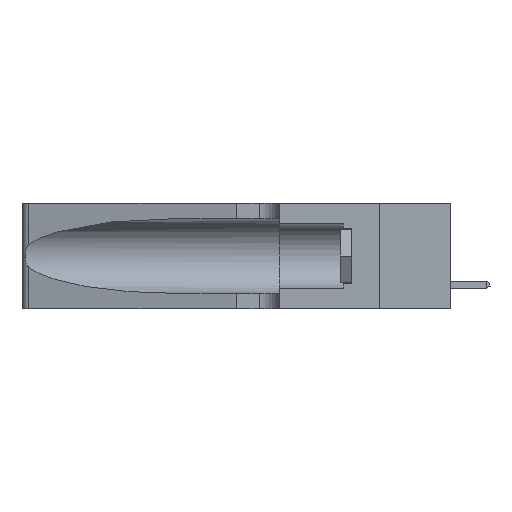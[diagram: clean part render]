
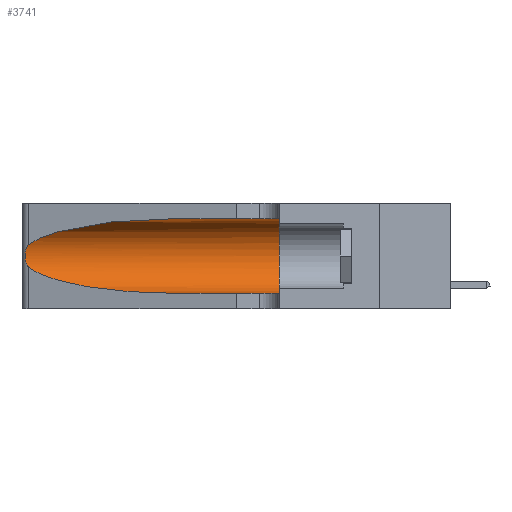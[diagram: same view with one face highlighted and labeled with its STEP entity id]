
A CAD part, left-side view. The second image highlights one B-rep face of the part: STEP entity #3741.
In plain terms, the highlighted cylindrical face has radius 3.308 mm (diameter 6.617 mm), a partial arc.
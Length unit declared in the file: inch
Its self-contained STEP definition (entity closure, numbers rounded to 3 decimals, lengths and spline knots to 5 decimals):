
#56 = CARTESIAN_POINT ( 'NONE',  ( 0.18966, 0.96281, 0.05475 ) ) ;
#865 = CARTESIAN_POINT ( 'NONE',  ( 0.26018, 1.23835, 0.19895 ) ) ;
#2405 = VERTEX_POINT ( 'NONE', #3868 ) ;
#3090 = VERTEX_POINT ( 'NONE', #22199 ) ;
#3415 = VERTEX_POINT ( 'NONE', #16453 ) ;
#3493 = CARTESIAN_POINT ( 'NONE',  ( 0.1305, 0.72297, 0.31525 ) ) ;
#3563 = EDGE_LOOP ( 'NONE', ( #20343, #20942, #22353, #11715, #9644, #24472 ) ) ;
#3741 = ADVANCED_FACE ( 'NONE', ( #6569 ), #15394, .F. ) ;
#3868 = CARTESIAN_POINT ( 'NONE',  ( 0.1305, 0.72297, 0.05475 ) ) ;
#3903 = CARTESIAN_POINT ( 'NONE',  ( 0.1305, 1.61858, 0.05475 ) ) ;
#4370 = CARTESIAN_POINT ( 'NONE',  ( 0.25787, 1.23484, 0.2124 ) ) ;
#4598 = DIRECTION ( 'NONE',  ( 0., -1., 0. ) ) ;
#4611 = VERTEX_POINT ( 'NONE', #9535 ) ;
#5170 = EDGE_CURVE ( 'NONE', #4611, #8581, #16346, .T. ) ;
#5773 = DIRECTION ( 'NONE',  ( 0., -1., 0. ) ) ;
#6014 = EDGE_CURVE ( 'NONE', #4611, #3415, #7759, .T. ) ;
#6287 = CARTESIAN_POINT ( 'NONE',  ( 0.25555, 1.22993, 0.14849 ) ) ;
#6569 = FACE_OUTER_BOUND ( 'NONE', #3563, .T. ) ;
#7571 = EDGE_CURVE ( 'NONE', #8581, #3090, #8627, .T. ) ;
#7658 = AXIS2_PLACEMENT_3D ( 'NONE', #19523, #15509, #13701 ) ;
#7759 = LINE ( 'NONE', #19672, #21714 ) ;
#7877 = CARTESIAN_POINT ( 'NONE',  ( 0.2373, 1.15595, 0.08982 ) ) ;
#8350 = CARTESIAN_POINT ( 'NONE',  ( 0.25854, 1.2359, 0.20912 ) ) ;
#8578 = CARTESIAN_POINT ( 'NONE',  ( 0.1305, 0.35, 0.185 ) ) ;
#8581 = VERTEX_POINT ( 'NONE', #15327 ) ;
#8627 = B_SPLINE_CURVE_WITH_KNOTS ( 'NONE', 3,
 ( #12137, #13804, #17693, #4370, #8350, #865, #23260, #11877, #17789, #10023, #13894, #19533, #6287, #10181 ),
 .UNSPECIFIED., .F., .F.,
 ( 4, 2, 2, 2, 2, 2, 4 ),
 ( 0., 0.00027, 0.00053, 0.00107, 0.0016, 0.00187, 0.00214 ),
 .UNSPECIFIED. ) ;
#8733 = DIRECTION ( 'NONE',  ( 0., 0., 1. ) ) ;
#9535 = CARTESIAN_POINT ( 'NONE',  ( 0.1305, 0.72297, 0.31525 ) ) ;
#9644 = ORIENTED_EDGE ( 'NONE', *, *, #20169, .F. ) ;
#10023 = CARTESIAN_POINT ( 'NONE',  ( 0.25856, 1.23593, 0.16098 ) ) ;
#10181 = CARTESIAN_POINT ( 'NONE',  ( 0.25487, 1.22718, 0.14631 ) ) ;
#10834 = EDGE_CURVE ( 'NONE', #3090, #2405, #15575, .T. ) ;
#11422 = EDGE_CURVE ( 'NONE', #2405, #16798, #13759, .T. ) ;
#11657 = CARTESIAN_POINT ( 'NONE',  ( 0.1305, 0.72297, 0.05475 ) ) ;
#11715 = ORIENTED_EDGE ( 'NONE', *, *, #11422, .T. ) ;
#11877 = CARTESIAN_POINT ( 'NONE',  ( 0.26075, 1.23896, 0.178 ) ) ;
#11966 = AXIS2_PLACEMENT_3D ( 'NONE', #8578, #12612, #8733 ) ;
#12137 = CARTESIAN_POINT ( 'NONE',  ( 0.25487, 1.22718, 0.22369 ) ) ;
#12612 = DIRECTION ( 'NONE',  ( 0., 1., 0. ) ) ;
#13701 = DIRECTION ( 'NONE',  ( 0., 0., -1. ) ) ;
#13759 = LINE ( 'NONE', #3903, #23540 ) ;
#13804 = CARTESIAN_POINT ( 'NONE',  ( 0.25555, 1.22994, 0.2215 ) ) ;
#13894 = CARTESIAN_POINT ( 'NONE',  ( 0.25789, 1.23486, 0.15765 ) ) ;
#15252 = CARTESIAN_POINT ( 'NONE',  ( 0.25487, 1.22718, 0.22369 ) ) ;
#15307 = CARTESIAN_POINT ( 'NONE',  ( 0.25487, 1.22718, 0.14631 ) ) ;
#15327 = CARTESIAN_POINT ( 'NONE',  ( 0.25487, 1.22718, 0.22369 ) ) ;
#15394 = CYLINDRICAL_SURFACE ( 'NONE', #7658, 0.13025 ) ;
#15423 = CARTESIAN_POINT ( 'NONE',  ( 0.2373, 1.15595, 0.28018 ) ) ;
#15509 = DIRECTION ( 'NONE',  ( 0., -1., 0. ) ) ;
#15575 =( BOUNDED_CURVE ( )  B_SPLINE_CURVE ( 3, ( #15307, #7877, #56, #11657 ),
 .UNSPECIFIED., .F., .T. ) 
 B_SPLINE_CURVE_WITH_KNOTS ( ( 4, 4 ),
 ( 3.44316, 4.71239 ),
 .UNSPECIFIED. ) 
 CURVE ( )  GEOMETRIC_REPRESENTATION_ITEM ( )  RATIONAL_B_SPLINE_CURVE ( ( 1., 0.87, 0.87, 1. ) ) 
 REPRESENTATION_ITEM ( '' )  );
#16346 =( BOUNDED_CURVE ( )  B_SPLINE_CURVE ( 3, ( #3493, #16770, #15423, #15252 ),
 .UNSPECIFIED., .F., .F. ) 
 B_SPLINE_CURVE_WITH_KNOTS ( ( 4, 4 ),
 ( 1.5708, 2.84003 ),
 .UNSPECIFIED. ) 
 CURVE ( )  GEOMETRIC_REPRESENTATION_ITEM ( )  RATIONAL_B_SPLINE_CURVE ( ( 1., 0.87, 0.87, 1. ) ) 
 REPRESENTATION_ITEM ( '' )  );
#16453 = CARTESIAN_POINT ( 'NONE',  ( 0.1305, 0.35, 0.31525 ) ) ;
#16770 = CARTESIAN_POINT ( 'NONE',  ( 0.18966, 0.96281, 0.31525 ) ) ;
#16798 = VERTEX_POINT ( 'NONE', #21925 ) ;
#17693 = CARTESIAN_POINT ( 'NONE',  ( 0.25639, 1.23184, 0.21858 ) ) ;
#17789 = CARTESIAN_POINT ( 'NONE',  ( 0.26017, 1.23833, 0.17102 ) ) ;
#19120 = CIRCLE ( 'NONE', #11966, 0.13025 ) ;
#19523 = CARTESIAN_POINT ( 'NONE',  ( 0.1305, 1.61858, 0.185 ) ) ;
#19533 = CARTESIAN_POINT ( 'NONE',  ( 0.25639, 1.23186, 0.15144 ) ) ;
#19672 = CARTESIAN_POINT ( 'NONE',  ( 0.1305, 1.61858, 0.31525 ) ) ;
#20169 = EDGE_CURVE ( 'NONE', #3415, #16798, #19120, .T. ) ;
#20343 = ORIENTED_EDGE ( 'NONE', *, *, #5170, .T. ) ;
#20942 = ORIENTED_EDGE ( 'NONE', *, *, #7571, .T. ) ;
#21714 = VECTOR ( 'NONE', #4598, 39.37008 ) ;
#21925 = CARTESIAN_POINT ( 'NONE',  ( 0.1305, 0.35, 0.05475 ) ) ;
#22199 = CARTESIAN_POINT ( 'NONE',  ( 0.25487, 1.22718, 0.14631 ) ) ;
#22353 = ORIENTED_EDGE ( 'NONE', *, *, #10834, .T. ) ;
#23260 = CARTESIAN_POINT ( 'NONE',  ( 0.26075, 1.23896, 0.19203 ) ) ;
#23540 = VECTOR ( 'NONE', #5773, 39.37008 ) ;
#24472 = ORIENTED_EDGE ( 'NONE', *, *, #6014, .F. ) ;
